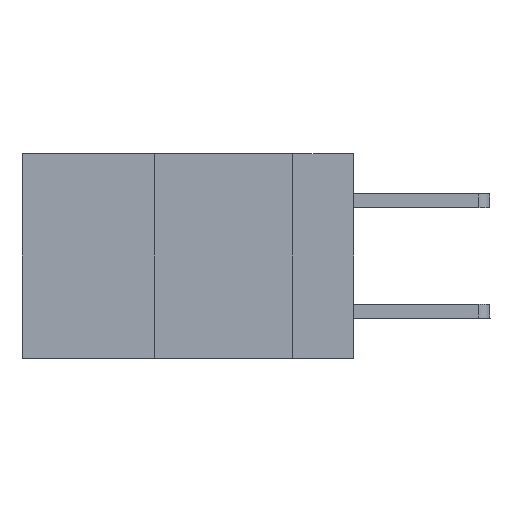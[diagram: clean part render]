
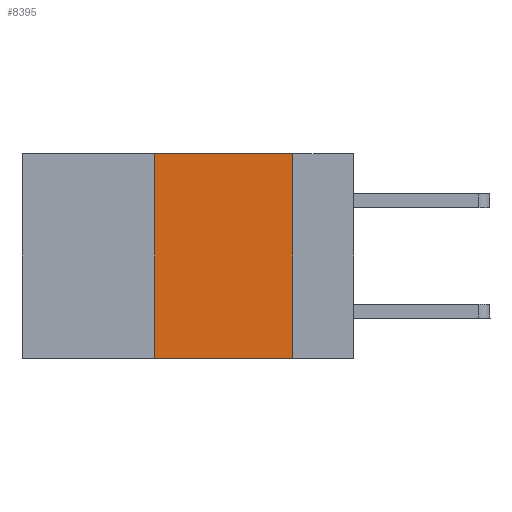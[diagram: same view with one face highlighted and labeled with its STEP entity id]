
A CAD part, left-side view. The second image highlights one B-rep face of the part: STEP entity #8395.
In plain terms, the highlighted planar face has unit normal (-1, 0, 0).
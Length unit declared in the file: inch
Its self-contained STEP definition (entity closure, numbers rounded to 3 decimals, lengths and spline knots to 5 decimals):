
#407 = EDGE_CURVE ( 'NONE', #6212, #522, #8082, .T. ) ;
#522 = VERTEX_POINT ( 'NONE', #6682 ) ;
#528 = CARTESIAN_POINT ( 'NONE',  ( 0., 0.6, 0. ) ) ;
#1137 = ORIENTED_EDGE ( 'NONE', *, *, #407, .F. ) ;
#1207 = ORIENTED_EDGE ( 'NONE', *, *, #9090, .T. ) ;
#1287 = ORIENTED_EDGE ( 'NONE', *, *, #4822, .F. ) ;
#1917 = CARTESIAN_POINT ( 'NONE',  ( 0., 0.36, 0. ) ) ;
#1995 = CARTESIAN_POINT ( 'NONE',  ( 0., 0.36, 0. ) ) ;
#2227 = LINE ( 'NONE', #9931, #8963 ) ;
#2501 = DIRECTION ( 'NONE',  ( 0., -1., 0. ) ) ;
#4157 = CARTESIAN_POINT ( 'NONE',  ( 0., 0.6, 0. ) ) ;
#4546 = DIRECTION ( 'NONE',  ( 0., -1., 0. ) ) ;
#4822 = EDGE_CURVE ( 'NONE', #5600, #10995, #7914, .T. ) ;
#5057 = DIRECTION ( 'NONE',  ( 0., 0., 1. ) ) ;
#5506 = VECTOR ( 'NONE', #5057, 39.37008 ) ;
#5600 = VERTEX_POINT ( 'NONE', #8807 ) ;
#5727 = LINE ( 'NONE', #4157, #10198 ) ;
#5940 = DIRECTION ( 'NONE',  ( 0., 0., -1. ) ) ;
#6212 = VERTEX_POINT ( 'NONE', #8556 ) ;
#6401 = ORIENTED_EDGE ( 'NONE', *, *, #7479, .F. ) ;
#6682 = CARTESIAN_POINT ( 'NONE',  ( 0., 0.11, -0.37 ) ) ;
#6810 = DIRECTION ( 'NONE',  ( 1., 0., 0. ) ) ;
#7345 = DIRECTION ( 'NONE',  ( 0., 0., -1. ) ) ;
#7479 = EDGE_CURVE ( 'NONE', #10995, #6212, #5727, .T. ) ;
#7502 = AXIS2_PLACEMENT_3D ( 'NONE', #528, #6810, #7345 ) ;
#7914 = LINE ( 'NONE', #1917, #5506 ) ;
#7947 = CARTESIAN_POINT ( 'NONE',  ( 0., 0.11, 0. ) ) ;
#8082 = LINE ( 'NONE', #7947, #10141 ) ;
#8179 = PLANE ( 'NONE',  #7502 ) ;
#8265 = FACE_OUTER_BOUND ( 'NONE', #9548, .T. ) ;
#8395 = ADVANCED_FACE ( 'NONE', ( #8265 ), #8179, .F. ) ;
#8556 = CARTESIAN_POINT ( 'NONE',  ( 0., 0.11, 0. ) ) ;
#8807 = CARTESIAN_POINT ( 'NONE',  ( 0., 0.36, -0.37 ) ) ;
#8963 = VECTOR ( 'NONE', #4546, 39.37008 ) ;
#9090 = EDGE_CURVE ( 'NONE', #5600, #522, #2227, .T. ) ;
#9548 = EDGE_LOOP ( 'NONE', ( #1137, #6401, #1287, #1207 ) ) ;
#9931 = CARTESIAN_POINT ( 'NONE',  ( 0., 0.6, -0.37 ) ) ;
#10141 = VECTOR ( 'NONE', #5940, 39.37008 ) ;
#10198 = VECTOR ( 'NONE', #2501, 39.37008 ) ;
#10995 = VERTEX_POINT ( 'NONE', #1995 ) ;
